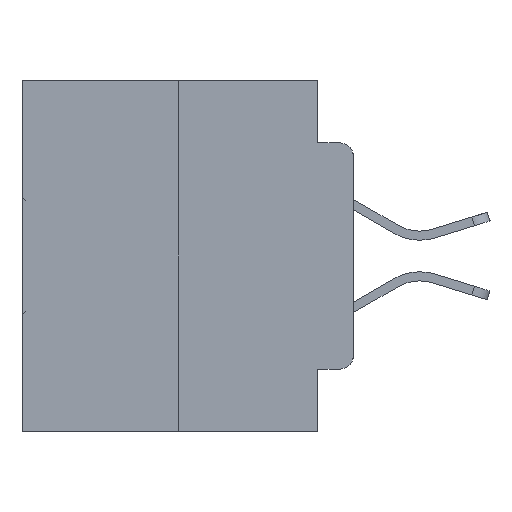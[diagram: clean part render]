
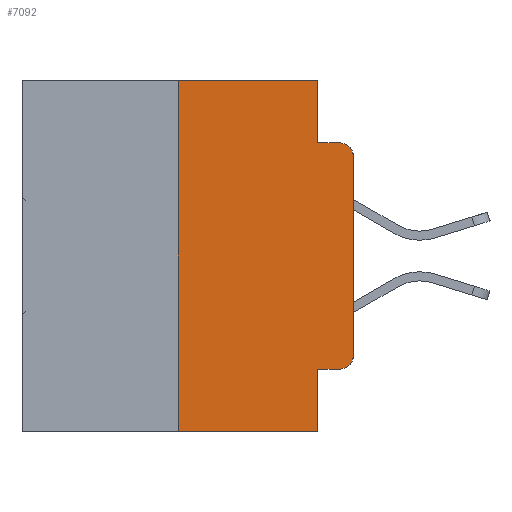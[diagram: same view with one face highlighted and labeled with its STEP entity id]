
A CAD part, left-side view. The second image highlights one B-rep face of the part: STEP entity #7092.
In plain terms, the highlighted planar face has unit normal (-1, 0, 0).
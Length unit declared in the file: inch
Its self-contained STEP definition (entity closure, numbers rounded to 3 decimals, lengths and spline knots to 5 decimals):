
#938 = DIRECTION ( 'NONE',  ( -1., 0., 0. ) ) ;
#1224 = VECTOR ( 'NONE', #27332, 39.37008 ) ;
#1801 = AXIS2_PLACEMENT_3D ( 'NONE', #15294, #32839, #17886 ) ;
#1872 = CARTESIAN_POINT ( 'NONE',  ( 0., 0., -0.1085 ) ) ;
#4000 = LINE ( 'NONE', #13200, #30151 ) ;
#4161 = FACE_OUTER_BOUND ( 'NONE', #30889, .T. ) ;
#4256 = CARTESIAN_POINT ( 'NONE',  ( 0., 0.051, 0. ) ) ;
#4971 = VECTOR ( 'NONE', #15878, 39.37008 ) ;
#5016 = VERTEX_POINT ( 'NONE', #16276 ) ;
#5611 = DIRECTION ( 'NONE',  ( 0., 0., -1. ) ) ;
#5894 = VERTEX_POINT ( 'NONE', #29866 ) ;
#6379 = VERTEX_POINT ( 'NONE', #1872 ) ;
#6706 = CARTESIAN_POINT ( 'NONE',  ( 0., 0.051, -0.0885 ) ) ;
#6843 = EDGE_CURVE ( 'NONE', #31214, #5016, #27203, .T. ) ;
#7081 = CARTESIAN_POINT ( 'NONE',  ( 0., 0.051, -0.4115 ) ) ;
#7092 = ADVANCED_FACE ( 'NONE', ( #4161 ), #9725, .F. ) ;
#7828 = VERTEX_POINT ( 'NONE', #32669 ) ;
#8264 = ORIENTED_EDGE ( 'NONE', *, *, #29495, .T. ) ;
#8483 = VECTOR ( 'NONE', #31552, 39.37008 ) ;
#8528 = EDGE_CURVE ( 'NONE', #22830, #27472, #27076, .T. ) ;
#8693 = CARTESIAN_POINT ( 'NONE',  ( 0., 0.25, 0. ) ) ;
#8884 = LINE ( 'NONE', #7081, #1224 ) ;
#9133 = LINE ( 'NONE', #14499, #28508 ) ;
#9725 = PLANE ( 'NONE',  #21727 ) ;
#10042 = CIRCLE ( 'NONE', #1801, 0.02 ) ;
#10273 = EDGE_CURVE ( 'NONE', #27472, #12843, #9133, .T. ) ;
#10750 = ORIENTED_EDGE ( 'NONE', *, *, #15364, .T. ) ;
#10776 = ORIENTED_EDGE ( 'NONE', *, *, #13656, .T. ) ;
#10780 = CARTESIAN_POINT ( 'NONE',  ( 0., 0.473, -0.5 ) ) ;
#11802 = LINE ( 'NONE', #10780, #4971 ) ;
#12413 = CARTESIAN_POINT ( 'NONE',  ( 0., 0.051, -0.4115 ) ) ;
#12843 = VERTEX_POINT ( 'NONE', #28017 ) ;
#13200 = CARTESIAN_POINT ( 'NONE',  ( 0., 0.051, 0. ) ) ;
#13656 = EDGE_CURVE ( 'NONE', #6379, #12843, #27188, .T. ) ;
#14242 = ORIENTED_EDGE ( 'NONE', *, *, #31147, .T. ) ;
#14499 = CARTESIAN_POINT ( 'NONE',  ( 0., 0.051, -0.0885 ) ) ;
#14817 = DIRECTION ( 'NONE',  ( 0., 0., -1. ) ) ;
#15268 = LINE ( 'NONE', #16554, #8483 ) ;
#15294 = CARTESIAN_POINT ( 'NONE',  ( 0., 0.02, -0.3915 ) ) ;
#15364 = EDGE_CURVE ( 'NONE', #5894, #6379, #16832, .T. ) ;
#15878 = DIRECTION ( 'NONE',  ( 0., -1., 0. ) ) ;
#16002 = ORIENTED_EDGE ( 'NONE', *, *, #6843, .F. ) ;
#16052 = CARTESIAN_POINT ( 'NONE',  ( 0., 0.051, -0.5 ) ) ;
#16276 = CARTESIAN_POINT ( 'NONE',  ( 0., 0.25, 0. ) ) ;
#16297 = CARTESIAN_POINT ( 'NONE',  ( 0., 0.02, -0.1085 ) ) ;
#16512 = ORIENTED_EDGE ( 'NONE', *, *, #26579, .T. ) ;
#16554 = CARTESIAN_POINT ( 'NONE',  ( 0., 0.473, 0. ) ) ;
#16640 = ORIENTED_EDGE ( 'NONE', *, *, #32812, .F. ) ;
#16832 = LINE ( 'NONE', #21268, #29402 ) ;
#17092 = DIRECTION ( 'NONE',  ( 0., -1., 0. ) ) ;
#17886 = DIRECTION ( 'NONE',  ( 0., 0., -1. ) ) ;
#18869 = DIRECTION ( 'NONE',  ( 0., 0., -1. ) ) ;
#20409 = DIRECTION ( 'NONE',  ( 0., 0., -1. ) ) ;
#21268 = CARTESIAN_POINT ( 'NONE',  ( 0., 0., 0. ) ) ;
#21727 = AXIS2_PLACEMENT_3D ( 'NONE', #27410, #29910, #14817 ) ;
#22830 = VERTEX_POINT ( 'NONE', #4256 ) ;
#22937 = CARTESIAN_POINT ( 'NONE',  ( 0., 0.051, 0. ) ) ;
#22940 = VERTEX_POINT ( 'NONE', #12413 ) ;
#23786 = DIRECTION ( 'NONE',  ( 0., 0., 1. ) ) ;
#24191 = AXIS2_PLACEMENT_3D ( 'NONE', #16297, #938, #18869 ) ;
#24703 = ORIENTED_EDGE ( 'NONE', *, *, #28684, .F. ) ;
#26579 = EDGE_CURVE ( 'NONE', #31214, #29680, #11802, .T. ) ;
#26835 = VECTOR ( 'NONE', #20409, 39.37008 ) ;
#27076 = LINE ( 'NONE', #22937, #26835 ) ;
#27188 = CIRCLE ( 'NONE', #24191, 0.02 ) ;
#27203 = LINE ( 'NONE', #8693, #31461 ) ;
#27332 = DIRECTION ( 'NONE',  ( 0., -1., 0. ) ) ;
#27410 = CARTESIAN_POINT ( 'NONE',  ( 0., 0.473, 0. ) ) ;
#27472 = VERTEX_POINT ( 'NONE', #6706 ) ;
#28017 = CARTESIAN_POINT ( 'NONE',  ( 0., 0.02, -0.0885 ) ) ;
#28162 = ORIENTED_EDGE ( 'NONE', *, *, #10273, .F. ) ;
#28508 = VECTOR ( 'NONE', #17092, 39.37008 ) ;
#28684 = EDGE_CURVE ( 'NONE', #5016, #22830, #15268, .T. ) ;
#28925 = DIRECTION ( 'NONE',  ( 0., 0., 1. ) ) ;
#29402 = VECTOR ( 'NONE', #23786, 39.37008 ) ;
#29495 = EDGE_CURVE ( 'NONE', #7828, #5894, #10042, .T. ) ;
#29680 = VERTEX_POINT ( 'NONE', #16052 ) ;
#29866 = CARTESIAN_POINT ( 'NONE',  ( 0., 0., -0.3915 ) ) ;
#29910 = DIRECTION ( 'NONE',  ( 1., 0., 0. ) ) ;
#30056 = CARTESIAN_POINT ( 'NONE',  ( 0., 0.25, -0.5 ) ) ;
#30151 = VECTOR ( 'NONE', #5611, 39.37008 ) ;
#30538 = ORIENTED_EDGE ( 'NONE', *, *, #8528, .F. ) ;
#30889 = EDGE_LOOP ( 'NONE', ( #10750, #10776, #28162, #30538, #24703, #16002, #16512, #16640, #14242, #8264 ) ) ;
#31147 = EDGE_CURVE ( 'NONE', #22940, #7828, #8884, .T. ) ;
#31214 = VERTEX_POINT ( 'NONE', #30056 ) ;
#31461 = VECTOR ( 'NONE', #28925, 39.37008 ) ;
#31552 = DIRECTION ( 'NONE',  ( 0., -1., 0. ) ) ;
#32669 = CARTESIAN_POINT ( 'NONE',  ( 0., 0.02, -0.4115 ) ) ;
#32812 = EDGE_CURVE ( 'NONE', #22940, #29680, #4000, .T. ) ;
#32839 = DIRECTION ( 'NONE',  ( -1., 0., 0. ) ) ;
